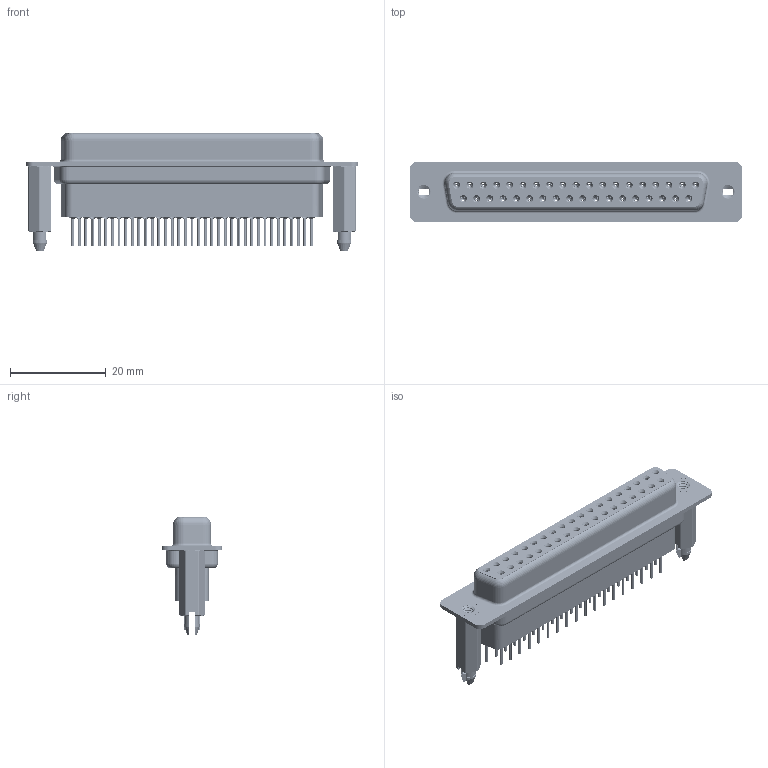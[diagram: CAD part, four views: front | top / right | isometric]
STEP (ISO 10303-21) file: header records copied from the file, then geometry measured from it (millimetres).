
FILE_DESCRIPTION (( 'STEP AP203' ), '1' );
FILE_NAME ('628-037-261-256.STEP', '2020-07-14T18:13:34', ( '' ), ( '' ), 'SwSTEP 2.0', 'SolidWorks 2020', '' );
FILE_SCHEMA (( 'CONFIG_CONTROL_DESIGN' ));
Length unit declared in the file: millimetre
Products named in the file (7): 628 Contact Row 2_61; 628-037-261-256; 628 Housing_37 HP; 628 Contact Row 1_61; 628 4-40 Threaded Boardlock_HP61; 628 Shell Rear_37 Contacts; 628 Shell Front_37 Contacts
Assembly tree (42 placements, depth 2):
  628-037-261-256
    628 Housing_37 HP
    628 Shell Front_37 Contacts
    628 Shell Rear_37 Contacts
    628 Contact Row 1_61  x19
    628 Contact Row 2_61  x18
    628 4-40 Threaded Boardlock_HP61  x2
Bounding box: 69.3 x 12.6 x 24.6 mm (x, y, z)
Volume: 7402.6 mm3; surface area: 16889.9 mm2
Topology: 42 solids, 42 shells, 4904 faces, 12609 edges, 7872 vertices
Faces by surface type: cylinder 1390, plane 1246, torus 951, bspline 746, cone 571
Entity records: 33752 total; most frequent: CARTESIAN_POINT 8782, DIRECTION 5168, ORIENTED_EDGE 4660, EDGE_CURVE 2330, AXIS2_PLACEMENT_3D 2165, VERTEX_POINT 1477, EDGE_LOOP 1191, CIRCLE 1179
